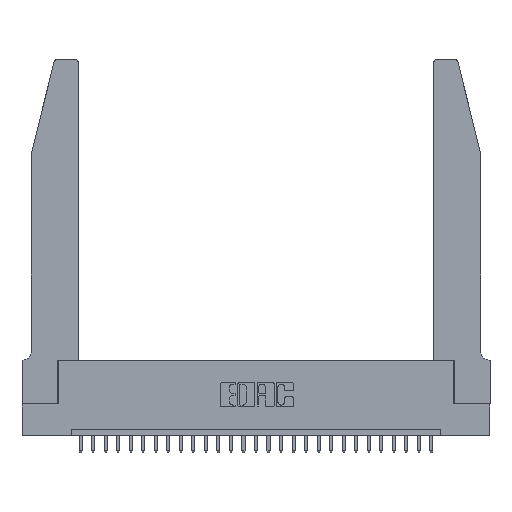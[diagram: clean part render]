
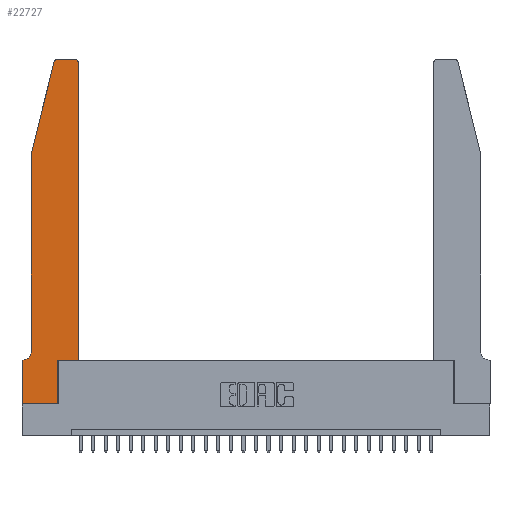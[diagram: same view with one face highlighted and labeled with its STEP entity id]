
A CAD part, top view. The second image highlights one B-rep face of the part: STEP entity #22727.
In plain terms, the highlighted planar face has unit normal (0, 0, 1).
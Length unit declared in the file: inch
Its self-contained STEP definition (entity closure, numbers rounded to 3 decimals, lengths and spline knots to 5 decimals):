
#213 = VECTOR ( 'NONE', #23079, 39.37008 ) ;
#471 = CARTESIAN_POINT ( 'NONE',  ( 0.284, 2.72, 0.37 ) ) ;
#1337 = CIRCLE ( 'NONE', #11158, 0.07 ) ;
#1731 = EDGE_CURVE ( 'NONE', #6462, #2252, #26373, .T. ) ;
#2049 = CARTESIAN_POINT ( 'NONE',  ( 0., 0.35, 0.37 ) ) ;
#2252 = VERTEX_POINT ( 'NONE', #22552 ) ;
#2577 = VECTOR ( 'NONE', #3033, 39.37008 ) ;
#3033 = DIRECTION ( 'NONE',  ( -0.239, -0.971, 0. ) ) ;
#3624 = DIRECTION ( 'NONE',  ( 1., 0., 0. ) ) ;
#3665 = EDGE_CURVE ( 'NONE', #4599, #6462, #13271, .T. ) ;
#3829 = CARTESIAN_POINT ( 'NONE',  ( 0., 0., 0.37 ) ) ;
#3981 = CIRCLE ( 'NONE', #14149, 0.03 ) ;
#4599 = VERTEX_POINT ( 'NONE', #21810 ) ;
#5067 = EDGE_CURVE ( 'NONE', #5628, #16957, #21780, .T. ) ;
#5491 = VECTOR ( 'NONE', #7556, 39.37008 ) ;
#5564 = CARTESIAN_POINT ( 'NONE',  ( 0.2865, 0.35, 0.37 ) ) ;
#5628 = VERTEX_POINT ( 'NONE', #12879 ) ;
#5756 = CARTESIAN_POINT ( 'NONE',  ( 0.0755, 0.35, 0.37 ) ) ;
#5812 = CARTESIAN_POINT ( 'NONE',  ( 0.0755, 2., 0.37 ) ) ;
#6238 = VECTOR ( 'NONE', #12862, 39.37008 ) ;
#6462 = VERTEX_POINT ( 'NONE', #21883 ) ;
#6494 = DIRECTION ( 'NONE',  ( -1., 0., 0. ) ) ;
#6567 = VECTOR ( 'NONE', #25465, 39.37008 ) ;
#6899 = DIRECTION ( 'NONE',  ( 0., 0., 1. ) ) ;
#7030 = VERTEX_POINT ( 'NONE', #13351 ) ;
#7152 = FACE_OUTER_BOUND ( 'NONE', #12226, .T. ) ;
#7208 = VERTEX_POINT ( 'NONE', #17395 ) ;
#7445 = ORIENTED_EDGE ( 'NONE', *, *, #10977, .T. ) ;
#7457 = ORIENTED_EDGE ( 'NONE', *, *, #23206, .T. ) ;
#7545 = ORIENTED_EDGE ( 'NONE', *, *, #14321, .T. ) ;
#7556 = DIRECTION ( 'NONE',  ( 1., 0., 0. ) ) ;
#7624 = ORIENTED_EDGE ( 'NONE', *, *, #16168, .T. ) ;
#7879 = EDGE_CURVE ( 'NONE', #13078, #4599, #9293, .T. ) ;
#8055 = CARTESIAN_POINT ( 'NONE',  ( 0., 0., 0.37 ) ) ;
#8815 = CARTESIAN_POINT ( 'NONE',  ( 0.0755, 2., 0.37 ) ) ;
#9293 = LINE ( 'NONE', #3829, #22337 ) ;
#9825 = CARTESIAN_POINT ( 'NONE',  ( 0.0755, 2., 0.37 ) ) ;
#10005 = ORIENTED_EDGE ( 'NONE', *, *, #5067, .T. ) ;
#10019 = CARTESIAN_POINT ( 'NONE',  ( 0.4505, 0.35, 0.37 ) ) ;
#10113 = DIRECTION ( 'NONE',  ( 0., 1., 0. ) ) ;
#10886 = CARTESIAN_POINT ( 'NONE',  ( 0.4505, 2.72, 0.37 ) ) ;
#10977 = EDGE_CURVE ( 'NONE', #7030, #18582, #12435, .T. ) ;
#11158 = AXIS2_PLACEMENT_3D ( 'NONE', #11537, #11733, #13741 ) ;
#11537 = CARTESIAN_POINT ( 'NONE',  ( 0.0055, 0.42, 0.37 ) ) ;
#11724 = AXIS2_PLACEMENT_3D ( 'NONE', #25698, #23614, #3624 ) ;
#11733 = DIRECTION ( 'NONE',  ( 0., 0., -1. ) ) ;
#11966 = ORIENTED_EDGE ( 'NONE', *, *, #1731, .T. ) ;
#12182 = ORIENTED_EDGE ( 'NONE', *, *, #7879, .T. ) ;
#12226 = EDGE_LOOP ( 'NONE', ( #7545, #10005, #23799, #27992, #7457, #7445, #7624, #12182, #15337, #11966, #21124, #13105 ) ) ;
#12298 = CARTESIAN_POINT ( 'NONE',  ( 0.25487, 2.72718, 0.37 ) ) ;
#12435 = LINE ( 'NONE', #5756, #6567 ) ;
#12862 = DIRECTION ( 'NONE',  ( 0., -1., 0. ) ) ;
#12879 = CARTESIAN_POINT ( 'NONE',  ( 0.284, 2.75, 0.37 ) ) ;
#13078 = VERTEX_POINT ( 'NONE', #25634 ) ;
#13105 = ORIENTED_EDGE ( 'NONE', *, *, #25707, .T. ) ;
#13271 = LINE ( 'NONE', #5564, #213 ) ;
#13351 = CARTESIAN_POINT ( 'NONE',  ( 0.0055, 0.35, 0.37 ) ) ;
#13741 = DIRECTION ( 'NONE',  ( -1., 0., 0. ) ) ;
#13858 = VECTOR ( 'NONE', #26355, 39.37008 ) ;
#14149 = AXIS2_PLACEMENT_3D ( 'NONE', #22659, #18566, #18665 ) ;
#14321 = EDGE_CURVE ( 'NONE', #7208, #5628, #18795, .T. ) ;
#14694 = VECTOR ( 'NONE', #6494, 39.37008 ) ;
#15337 = ORIENTED_EDGE ( 'NONE', *, *, #3665, .T. ) ;
#15598 = LINE ( 'NONE', #8815, #13858 ) ;
#16168 = EDGE_CURVE ( 'NONE', #18582, #13078, #24371, .T. ) ;
#16957 = VERTEX_POINT ( 'NONE', #12298 ) ;
#17395 = CARTESIAN_POINT ( 'NONE',  ( 0.4205, 2.75, 0.37 ) ) ;
#17948 = DIRECTION ( 'NONE',  ( 1., 0., 0. ) ) ;
#18536 = VERTEX_POINT ( 'NONE', #21613 ) ;
#18566 = DIRECTION ( 'NONE',  ( 0., 0., 1. ) ) ;
#18582 = VERTEX_POINT ( 'NONE', #2049 ) ;
#18665 = DIRECTION ( 'NONE',  ( 1., 0., 0. ) ) ;
#18795 = LINE ( 'NONE', #19816, #14694 ) ;
#18973 = VERTEX_POINT ( 'NONE', #10886 ) ;
#19816 = CARTESIAN_POINT ( 'NONE',  ( 0.2605, 2.75, 0.37 ) ) ;
#20227 = EDGE_CURVE ( 'NONE', #2252, #18973, #20790, .T. ) ;
#20790 = LINE ( 'NONE', #10019, #22456 ) ;
#20865 = PLANE ( 'NONE',  #11724 ) ;
#21124 = ORIENTED_EDGE ( 'NONE', *, *, #20227, .T. ) ;
#21613 = CARTESIAN_POINT ( 'NONE',  ( 0.0755, 0.42, 0.37 ) ) ;
#21620 = VERTEX_POINT ( 'NONE', #5812 ) ;
#21780 = CIRCLE ( 'NONE', #22016, 0.03 ) ;
#21805 = LINE ( 'NONE', #9825, #2577 ) ;
#21810 = CARTESIAN_POINT ( 'NONE',  ( 0.2865, 0., 0.37 ) ) ;
#21883 = CARTESIAN_POINT ( 'NONE',  ( 0.2865, 0.35, 0.37 ) ) ;
#22016 = AXIS2_PLACEMENT_3D ( 'NONE', #471, #6899, #17948 ) ;
#22337 = VECTOR ( 'NONE', #27910, 39.37008 ) ;
#22456 = VECTOR ( 'NONE', #10113, 39.37008 ) ;
#22552 = CARTESIAN_POINT ( 'NONE',  ( 0.4505, 0.35, 0.37 ) ) ;
#22659 = CARTESIAN_POINT ( 'NONE',  ( 0.4205, 2.72, 0.37 ) ) ;
#22727 = ADVANCED_FACE ( 'NONE', ( #7152 ), #20865, .T. ) ;
#22809 = CARTESIAN_POINT ( 'NONE',  ( 0.4505, 0.35, 0.37 ) ) ;
#23079 = DIRECTION ( 'NONE',  ( 0., 1., 0. ) ) ;
#23206 = EDGE_CURVE ( 'NONE', #18536, #7030, #1337, .T. ) ;
#23614 = DIRECTION ( 'NONE',  ( 0., 0., 1. ) ) ;
#23799 = ORIENTED_EDGE ( 'NONE', *, *, #25748, .T. ) ;
#24371 = LINE ( 'NONE', #8055, #6238 ) ;
#25465 = DIRECTION ( 'NONE',  ( -1., 0., 0. ) ) ;
#25634 = CARTESIAN_POINT ( 'NONE',  ( 0., 0., 0.37 ) ) ;
#25698 = CARTESIAN_POINT ( 'NONE',  ( 0., 0.35, 0.37 ) ) ;
#25707 = EDGE_CURVE ( 'NONE', #18973, #7208, #3981, .T. ) ;
#25748 = EDGE_CURVE ( 'NONE', #16957, #21620, #21805, .T. ) ;
#26146 = EDGE_CURVE ( 'NONE', #21620, #18536, #15598, .T. ) ;
#26355 = DIRECTION ( 'NONE',  ( 0., -1., 0. ) ) ;
#26373 = LINE ( 'NONE', #22809, #5491 ) ;
#27910 = DIRECTION ( 'NONE',  ( 1., 0., 0. ) ) ;
#27992 = ORIENTED_EDGE ( 'NONE', *, *, #26146, .T. ) ;
